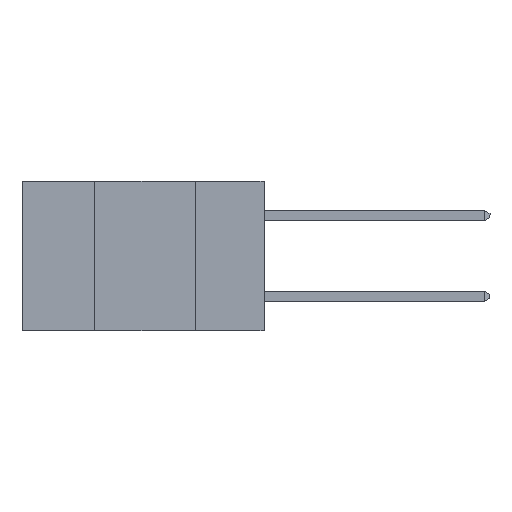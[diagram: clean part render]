
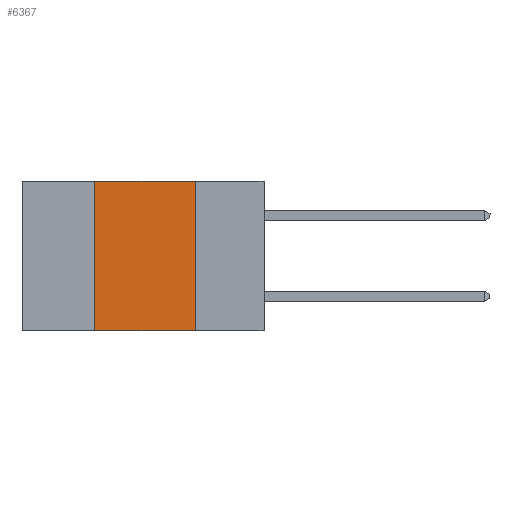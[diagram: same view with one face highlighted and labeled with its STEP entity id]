
A CAD part, left-side view. The second image highlights one B-rep face of the part: STEP entity #6367.
In plain terms, the highlighted planar face has unit normal (-1, 0, 0).
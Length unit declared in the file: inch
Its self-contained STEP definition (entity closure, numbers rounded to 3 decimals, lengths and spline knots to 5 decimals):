
#632 = VERTEX_POINT ( 'NONE', #15073 ) ;
#908 = ORIENTED_EDGE ( 'NONE', *, *, #8904, .F. ) ;
#1395 = VERTEX_POINT ( 'NONE', #4542 ) ;
#1588 = VERTEX_POINT ( 'NONE', #4991 ) ;
#2257 = AXIS2_PLACEMENT_3D ( 'NONE', #9929, #4997, #13535 ) ;
#2664 = DIRECTION ( 'NONE',  ( 0., 0., 1. ) ) ;
#2776 = VECTOR ( 'NONE', #2664, 39.37008 ) ;
#3045 = VECTOR ( 'NONE', #5505, 39.37008 ) ;
#4246 = VECTOR ( 'NONE', #6901, 39.37008 ) ;
#4486 = EDGE_CURVE ( 'NONE', #1395, #1588, #12526, .T. ) ;
#4542 = CARTESIAN_POINT ( 'NONE',  ( 0., 0.42, -0.37 ) ) ;
#4991 = CARTESIAN_POINT ( 'NONE',  ( 0., 0.17, -0.37 ) ) ;
#4997 = DIRECTION ( 'NONE',  ( 1., 0., 0. ) ) ;
#5505 = DIRECTION ( 'NONE',  ( 0., -1., 0. ) ) ;
#5635 = CARTESIAN_POINT ( 'NONE',  ( 0., 0.17, 0. ) ) ;
#5878 = EDGE_CURVE ( 'NONE', #1395, #632, #15233, .T. ) ;
#6038 = VECTOR ( 'NONE', #14099, 39.37008 ) ;
#6334 = LINE ( 'NONE', #10442, #3045 ) ;
#6367 = ADVANCED_FACE ( 'NONE', ( #8945 ), #8699, .F. ) ;
#6725 = EDGE_CURVE ( 'NONE', #9540, #1588, #10833, .T. ) ;
#6901 = DIRECTION ( 'NONE',  ( 0., 0., -1. ) ) ;
#8141 = ORIENTED_EDGE ( 'NONE', *, *, #6725, .F. ) ;
#8355 = ORIENTED_EDGE ( 'NONE', *, *, #5878, .F. ) ;
#8549 = EDGE_LOOP ( 'NONE', ( #8141, #908, #8355, #8762 ) ) ;
#8699 = PLANE ( 'NONE',  #2257 ) ;
#8762 = ORIENTED_EDGE ( 'NONE', *, *, #4486, .T. ) ;
#8824 = CARTESIAN_POINT ( 'NONE',  ( 0., 0.42, 0. ) ) ;
#8904 = EDGE_CURVE ( 'NONE', #632, #9540, #6334, .T. ) ;
#8945 = FACE_OUTER_BOUND ( 'NONE', #8549, .T. ) ;
#9540 = VERTEX_POINT ( 'NONE', #13843 ) ;
#9929 = CARTESIAN_POINT ( 'NONE',  ( 0., 0.6, 0. ) ) ;
#10442 = CARTESIAN_POINT ( 'NONE',  ( 0., 0.6, 0. ) ) ;
#10833 = LINE ( 'NONE', #5635, #4246 ) ;
#12526 = LINE ( 'NONE', #13649, #6038 ) ;
#13535 = DIRECTION ( 'NONE',  ( 0., 0., -1. ) ) ;
#13649 = CARTESIAN_POINT ( 'NONE',  ( 0., 0.6, -0.37 ) ) ;
#13843 = CARTESIAN_POINT ( 'NONE',  ( 0., 0.17, 0. ) ) ;
#14099 = DIRECTION ( 'NONE',  ( 0., -1., 0. ) ) ;
#15073 = CARTESIAN_POINT ( 'NONE',  ( 0., 0.42, 0. ) ) ;
#15233 = LINE ( 'NONE', #8824, #2776 ) ;
